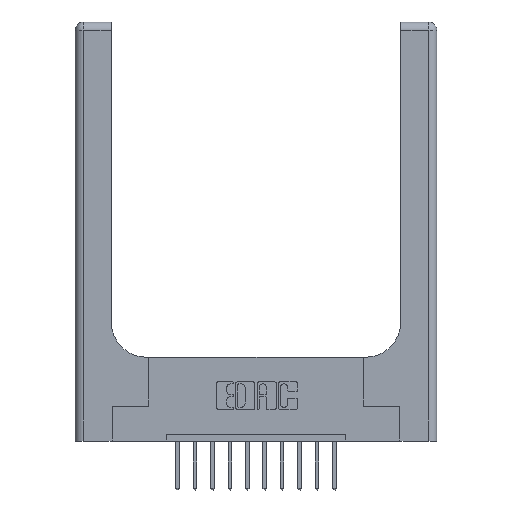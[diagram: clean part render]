
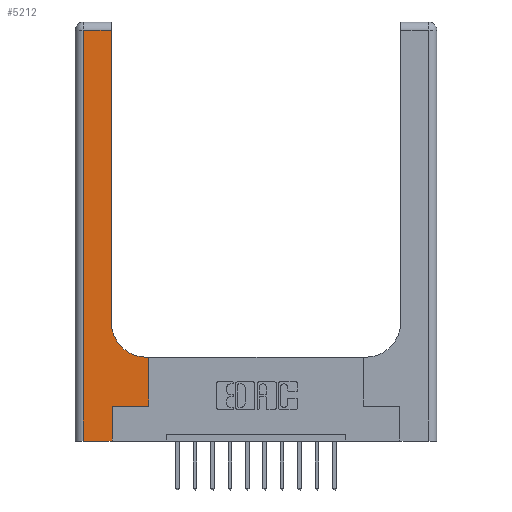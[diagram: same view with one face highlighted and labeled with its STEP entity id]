
A CAD part, top view. The second image highlights one B-rep face of the part: STEP entity #5212.
In plain terms, the highlighted planar face has unit normal (0, 0, 1).
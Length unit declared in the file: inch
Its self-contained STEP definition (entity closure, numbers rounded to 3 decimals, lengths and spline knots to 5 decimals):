
#376 = CARTESIAN_POINT ( 'NONE',  ( 0.265, 0., 0.37 ) ) ;
#615 = EDGE_CURVE ( 'NONE', #14398, #2153, #11066, .T. ) ;
#745 = FACE_OUTER_BOUND ( 'NONE', #1018, .T. ) ;
#839 = VECTOR ( 'NONE', #15076, 39.37008 ) ;
#1018 = EDGE_LOOP ( 'NONE', ( #15753, #2496, #15394, #12325, #7415, #9870, #15665, #4099, #9644 ) ) ;
#1668 = DIRECTION ( 'NONE',  ( 0., 1., 0. ) ) ;
#1714 = LINE ( 'NONE', #14408, #9094 ) ;
#1775 = VECTOR ( 'NONE', #14424, 39.37008 ) ;
#1870 = CARTESIAN_POINT ( 'NONE',  ( 0.51, 0.85, 0.37 ) ) ;
#2087 = VERTEX_POINT ( 'NONE', #2743 ) ;
#2149 = VECTOR ( 'NONE', #1668, 39.37008 ) ;
#2153 = VERTEX_POINT ( 'NONE', #11417 ) ;
#2462 = CARTESIAN_POINT ( 'NONE',  ( 0.265, 0., 0.37 ) ) ;
#2496 = ORIENTED_EDGE ( 'NONE', *, *, #10419, .T. ) ;
#2743 = CARTESIAN_POINT ( 'NONE',  ( 0.26, 2.94, 0.37 ) ) ;
#2910 = DIRECTION ( 'NONE',  ( 1., 0., 0. ) ) ;
#3360 = VERTEX_POINT ( 'NONE', #4177 ) ;
#3642 = LINE ( 'NONE', #7560, #11519 ) ;
#4099 = ORIENTED_EDGE ( 'NONE', *, *, #4892, .T. ) ;
#4177 = CARTESIAN_POINT ( 'NONE',  ( 0.528, 0.25, 0.37 ) ) ;
#4220 = EDGE_CURVE ( 'NONE', #14787, #3360, #9105, .T. ) ;
#4250 = LINE ( 'NONE', #10386, #1775 ) ;
#4476 = DIRECTION ( 'NONE',  ( -1., 0., 0. ) ) ;
#4534 = VERTEX_POINT ( 'NONE', #2462 ) ;
#4892 = EDGE_CURVE ( 'NONE', #10950, #14398, #14879, .T. ) ;
#5212 = ADVANCED_FACE ( 'NONE', ( #745 ), #5768, .F. ) ;
#5265 = EDGE_CURVE ( 'NONE', #3360, #10950, #3642, .T. ) ;
#5768 = PLANE ( 'NONE',  #12831 ) ;
#5931 = CARTESIAN_POINT ( 'NONE',  ( 0.265, 0.25, 0.37 ) ) ;
#6361 = CARTESIAN_POINT ( 'NONE',  ( 0.06, 2.94, 0.37 ) ) ;
#6665 = DIRECTION ( 'NONE',  ( 0., 1., 0. ) ) ;
#6762 = DIRECTION ( 'NONE',  ( -1., 0., 0. ) ) ;
#6874 = LINE ( 'NONE', #376, #2149 ) ;
#7177 = EDGE_CURVE ( 'NONE', #4534, #14787, #6874, .T. ) ;
#7260 = DIRECTION ( 'NONE',  ( -1., 0., 0. ) ) ;
#7415 = ORIENTED_EDGE ( 'NONE', *, *, #7177, .T. ) ;
#7560 = CARTESIAN_POINT ( 'NONE',  ( 0.528, 0.25, 0.37 ) ) ;
#8002 = CARTESIAN_POINT ( 'NONE',  ( 0., 2.94, 0.37 ) ) ;
#8426 = CARTESIAN_POINT ( 'NONE',  ( 0.51, 0.6, 0.37 ) ) ;
#8681 = VERTEX_POINT ( 'NONE', #6361 ) ;
#9094 = VECTOR ( 'NONE', #6665, 39.37008 ) ;
#9105 = LINE ( 'NONE', #14133, #12529 ) ;
#9115 = CARTESIAN_POINT ( 'NONE',  ( 0.06, 0., 0.37 ) ) ;
#9220 = LINE ( 'NONE', #8002, #14804 ) ;
#9456 = DIRECTION ( 'NONE',  ( 1., 0., 0. ) ) ;
#9569 = VERTEX_POINT ( 'NONE', #9115 ) ;
#9644 = ORIENTED_EDGE ( 'NONE', *, *, #615, .T. ) ;
#9870 = ORIENTED_EDGE ( 'NONE', *, *, #4220, .T. ) ;
#9878 = CARTESIAN_POINT ( 'NONE',  ( 0.26, 0.6, 0.37 ) ) ;
#9944 = DIRECTION ( 'NONE',  ( 0., 1., 0. ) ) ;
#10386 = CARTESIAN_POINT ( 'NONE',  ( 0.06, 3., 0.37 ) ) ;
#10419 = EDGE_CURVE ( 'NONE', #2087, #8681, #9220, .T. ) ;
#10950 = VERTEX_POINT ( 'NONE', #15572 ) ;
#11066 = CIRCLE ( 'NONE', #14966, 0.25 ) ;
#11282 = EDGE_CURVE ( 'NONE', #9569, #4534, #13709, .T. ) ;
#11417 = CARTESIAN_POINT ( 'NONE',  ( 0.26, 0.85, 0.37 ) ) ;
#11519 = VECTOR ( 'NONE', #9944, 39.37008 ) ;
#11860 = DIRECTION ( 'NONE',  ( 0., 0., -1. ) ) ;
#12325 = ORIENTED_EDGE ( 'NONE', *, *, #11282, .T. ) ;
#12404 = CARTESIAN_POINT ( 'NONE',  ( 0., 0., 0.37 ) ) ;
#12529 = VECTOR ( 'NONE', #2910, 39.37008 ) ;
#12831 = AXIS2_PLACEMENT_3D ( 'NONE', #14551, #11860, #4476 ) ;
#13022 = EDGE_CURVE ( 'NONE', #8681, #9569, #4250, .T. ) ;
#13709 = LINE ( 'NONE', #12404, #839 ) ;
#13859 = VECTOR ( 'NONE', #7260, 39.37008 ) ;
#14133 = CARTESIAN_POINT ( 'NONE',  ( 0.265, 0.25, 0.37 ) ) ;
#14398 = VERTEX_POINT ( 'NONE', #8426 ) ;
#14408 = CARTESIAN_POINT ( 'NONE',  ( 0.26, 3., 0.37 ) ) ;
#14424 = DIRECTION ( 'NONE',  ( 0., -1., 0. ) ) ;
#14551 = CARTESIAN_POINT ( 'NONE',  ( 0., 3., 0.37 ) ) ;
#14647 = EDGE_CURVE ( 'NONE', #2153, #2087, #1714, .T. ) ;
#14787 = VERTEX_POINT ( 'NONE', #5931 ) ;
#14804 = VECTOR ( 'NONE', #6762, 39.37008 ) ;
#14879 = LINE ( 'NONE', #9878, #13859 ) ;
#14966 = AXIS2_PLACEMENT_3D ( 'NONE', #1870, #15591, #9456 ) ;
#15076 = DIRECTION ( 'NONE',  ( 1., 0., 0. ) ) ;
#15394 = ORIENTED_EDGE ( 'NONE', *, *, #13022, .T. ) ;
#15572 = CARTESIAN_POINT ( 'NONE',  ( 0.528, 0.6, 0.37 ) ) ;
#15591 = DIRECTION ( 'NONE',  ( 0., 0., -1. ) ) ;
#15665 = ORIENTED_EDGE ( 'NONE', *, *, #5265, .T. ) ;
#15753 = ORIENTED_EDGE ( 'NONE', *, *, #14647, .T. ) ;
